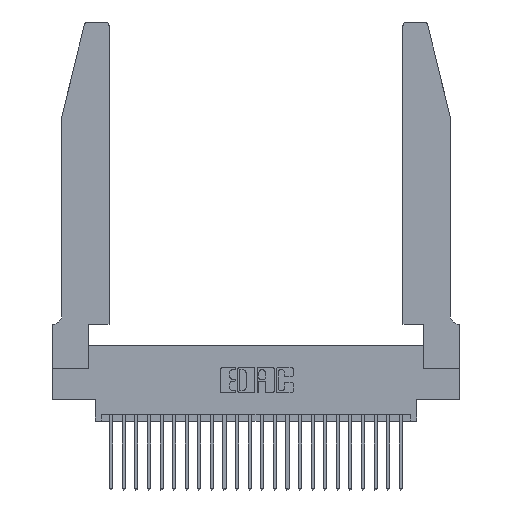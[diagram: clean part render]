
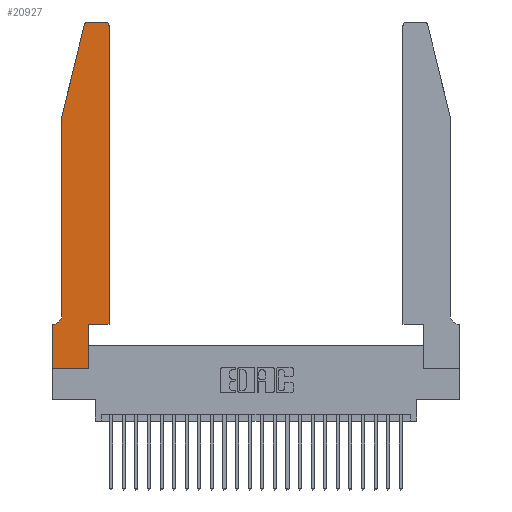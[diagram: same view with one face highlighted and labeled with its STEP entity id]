
A CAD part, top view. The second image highlights one B-rep face of the part: STEP entity #20927.
In plain terms, the highlighted planar face has unit normal (0, 0, 1).
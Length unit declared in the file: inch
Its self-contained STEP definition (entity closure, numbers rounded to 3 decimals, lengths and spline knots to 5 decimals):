
#40 = DIRECTION ( 'NONE',  ( 1., 0., 0. ) ) ;
#59 = EDGE_CURVE ( 'NONE', #6156, #24500, #25750, .T. ) ;
#77 = CARTESIAN_POINT ( 'NONE',  ( 0.2865, 0.35, 0.37 ) ) ;
#344 = DIRECTION ( 'NONE',  ( 0., 1., 0. ) ) ;
#555 = ORIENTED_EDGE ( 'NONE', *, *, #59, .T. ) ;
#828 = VERTEX_POINT ( 'NONE', #5476 ) ;
#865 = AXIS2_PLACEMENT_3D ( 'NONE', #5088, #19230, #7171 ) ;
#963 = VERTEX_POINT ( 'NONE', #14383 ) ;
#1056 = ORIENTED_EDGE ( 'NONE', *, *, #15632, .T. ) ;
#1144 = VECTOR ( 'NONE', #11737, 39.37008 ) ;
#1165 = LINE ( 'NONE', #24578, #11424 ) ;
#1598 = EDGE_CURVE ( 'NONE', #7132, #828, #25560, .T. ) ;
#1786 = VECTOR ( 'NONE', #26148, 39.37008 ) ;
#2011 = CARTESIAN_POINT ( 'NONE',  ( 0.0755, 2., 0.37 ) ) ;
#2216 = ORIENTED_EDGE ( 'NONE', *, *, #18495, .T. ) ;
#3064 = CARTESIAN_POINT ( 'NONE',  ( 0.284, 2.75, 0.37 ) ) ;
#3871 = EDGE_CURVE ( 'NONE', #4540, #17209, #17998, .T. ) ;
#3935 = CARTESIAN_POINT ( 'NONE',  ( 0., 0.35, 0.37 ) ) ;
#3973 = ORIENTED_EDGE ( 'NONE', *, *, #9391, .T. ) ;
#4165 = VERTEX_POINT ( 'NONE', #3064 ) ;
#4263 = FACE_OUTER_BOUND ( 'NONE', #11685, .T. ) ;
#4540 = VERTEX_POINT ( 'NONE', #16641 ) ;
#4904 = LINE ( 'NONE', #23751, #15704 ) ;
#4989 = CARTESIAN_POINT ( 'NONE',  ( 0.4205, 2.72, 0.37 ) ) ;
#5088 = CARTESIAN_POINT ( 'NONE',  ( 0.0055, 0.42, 0.37 ) ) ;
#5476 = CARTESIAN_POINT ( 'NONE',  ( 0.4505, 0.35, 0.37 ) ) ;
#5814 = CARTESIAN_POINT ( 'NONE',  ( 0.2865, 0.35, 0.37 ) ) ;
#5898 = CIRCLE ( 'NONE', #865, 0.07 ) ;
#6156 = VERTEX_POINT ( 'NONE', #20786 ) ;
#6157 = VECTOR ( 'NONE', #11279, 39.37008 ) ;
#6545 = ORIENTED_EDGE ( 'NONE', *, *, #12373, .T. ) ;
#6580 = CARTESIAN_POINT ( 'NONE',  ( 0.0755, 0.42, 0.37 ) ) ;
#6770 = CARTESIAN_POINT ( 'NONE',  ( 0.0755, 2., 0.37 ) ) ;
#7082 = DIRECTION ( 'NONE',  ( 1., 0., 0. ) ) ;
#7125 = DIRECTION ( 'NONE',  ( 0., -1., 0. ) ) ;
#7132 = VERTEX_POINT ( 'NONE', #5814 ) ;
#7171 = DIRECTION ( 'NONE',  ( -1., 0., 0. ) ) ;
#7300 = EDGE_CURVE ( 'NONE', #4165, #4540, #15929, .T. ) ;
#7545 = ORIENTED_EDGE ( 'NONE', *, *, #11584, .T. ) ;
#7758 = DIRECTION ( 'NONE',  ( -1., 0., 0. ) ) ;
#7965 = CARTESIAN_POINT ( 'NONE',  ( 0.4505, 0.35, 0.37 ) ) ;
#8143 = CARTESIAN_POINT ( 'NONE',  ( 0., 0., 0.37 ) ) ;
#8240 = ORIENTED_EDGE ( 'NONE', *, *, #1598, .T. ) ;
#8410 = DIRECTION ( 'NONE',  ( 0., 0., 1. ) ) ;
#8808 = VERTEX_POINT ( 'NONE', #15715 ) ;
#9036 = EDGE_CURVE ( 'NONE', #24500, #7132, #14910, .T. ) ;
#9258 = CARTESIAN_POINT ( 'NONE',  ( 0.2605, 2.75, 0.37 ) ) ;
#9391 = EDGE_CURVE ( 'NONE', #22460, #6156, #22685, .T. ) ;
#9903 = AXIS2_PLACEMENT_3D ( 'NONE', #20460, #8410, #22458 ) ;
#10025 = DIRECTION ( 'NONE',  ( 1., 0., 0. ) ) ;
#10163 = VECTOR ( 'NONE', #14414, 39.37008 ) ;
#11210 = CARTESIAN_POINT ( 'NONE',  ( 0.0755, 2., 0.37 ) ) ;
#11279 = DIRECTION ( 'NONE',  ( -1., 0., 0. ) ) ;
#11424 = VECTOR ( 'NONE', #344, 39.37008 ) ;
#11584 = EDGE_CURVE ( 'NONE', #19014, #8808, #5898, .T. ) ;
#11685 = EDGE_LOOP ( 'NONE', ( #14096, #15001, #23433, #1056, #7545, #6545, #3973, #555, #21401, #8240, #13299, #2216 ) ) ;
#11737 = DIRECTION ( 'NONE',  ( 0., -1., 0. ) ) ;
#12262 = LINE ( 'NONE', #11210, #22262 ) ;
#12373 = EDGE_CURVE ( 'NONE', #8808, #22460, #4904, .T. ) ;
#12774 = EDGE_CURVE ( 'NONE', #963, #4165, #16946, .T. ) ;
#13299 = ORIENTED_EDGE ( 'NONE', *, *, #24487, .T. ) ;
#14096 = ORIENTED_EDGE ( 'NONE', *, *, #12774, .T. ) ;
#14207 = DIRECTION ( 'NONE',  ( 1., 0., 0. ) ) ;
#14383 = CARTESIAN_POINT ( 'NONE',  ( 0.4205, 2.75, 0.37 ) ) ;
#14414 = DIRECTION ( 'NONE',  ( 0., 1., 0. ) ) ;
#14910 = LINE ( 'NONE', #77, #10163 ) ;
#15001 = ORIENTED_EDGE ( 'NONE', *, *, #7300, .T. ) ;
#15632 = EDGE_CURVE ( 'NONE', #17209, #19014, #12262, .T. ) ;
#15704 = VECTOR ( 'NONE', #7758, 39.37008 ) ;
#15715 = CARTESIAN_POINT ( 'NONE',  ( 0.0055, 0.35, 0.37 ) ) ;
#15853 = AXIS2_PLACEMENT_3D ( 'NONE', #3935, #26097, #14207 ) ;
#15929 = CIRCLE ( 'NONE', #9903, 0.03 ) ;
#15949 = VERTEX_POINT ( 'NONE', #22316 ) ;
#16048 = CARTESIAN_POINT ( 'NONE',  ( 0., 0.35, 0.37 ) ) ;
#16641 = CARTESIAN_POINT ( 'NONE',  ( 0.25487, 2.72718, 0.37 ) ) ;
#16946 = LINE ( 'NONE', #9258, #6157 ) ;
#17209 = VERTEX_POINT ( 'NONE', #6770 ) ;
#17998 = LINE ( 'NONE', #2011, #1786 ) ;
#18000 = AXIS2_PLACEMENT_3D ( 'NONE', #4989, #19143, #7082 ) ;
#18495 = EDGE_CURVE ( 'NONE', #15949, #963, #19623, .T. ) ;
#19014 = VERTEX_POINT ( 'NONE', #6580 ) ;
#19143 = DIRECTION ( 'NONE',  ( 0., 0., 1. ) ) ;
#19230 = DIRECTION ( 'NONE',  ( 0., 0., -1. ) ) ;
#19623 = CIRCLE ( 'NONE', #18000, 0.03 ) ;
#20120 = PLANE ( 'NONE',  #15853 ) ;
#20296 = VECTOR ( 'NONE', #40, 39.37008 ) ;
#20460 = CARTESIAN_POINT ( 'NONE',  ( 0.284, 2.72, 0.37 ) ) ;
#20487 = VECTOR ( 'NONE', #10025, 39.37008 ) ;
#20675 = CARTESIAN_POINT ( 'NONE',  ( 0.2865, 0., 0.37 ) ) ;
#20786 = CARTESIAN_POINT ( 'NONE',  ( 0., 0., 0.37 ) ) ;
#20927 = ADVANCED_FACE ( 'NONE', ( #4263 ), #20120, .T. ) ;
#21401 = ORIENTED_EDGE ( 'NONE', *, *, #9036, .T. ) ;
#21731 = CARTESIAN_POINT ( 'NONE',  ( 0., 0., 0.37 ) ) ;
#22262 = VECTOR ( 'NONE', #7125, 39.37008 ) ;
#22316 = CARTESIAN_POINT ( 'NONE',  ( 0.4505, 2.72, 0.37 ) ) ;
#22458 = DIRECTION ( 'NONE',  ( 1., 0., 0. ) ) ;
#22460 = VERTEX_POINT ( 'NONE', #16048 ) ;
#22685 = LINE ( 'NONE', #21731, #1144 ) ;
#23433 = ORIENTED_EDGE ( 'NONE', *, *, #3871, .T. ) ;
#23751 = CARTESIAN_POINT ( 'NONE',  ( 0.0755, 0.35, 0.37 ) ) ;
#24487 = EDGE_CURVE ( 'NONE', #828, #15949, #1165, .T. ) ;
#24500 = VERTEX_POINT ( 'NONE', #20675 ) ;
#24578 = CARTESIAN_POINT ( 'NONE',  ( 0.4505, 0.35, 0.37 ) ) ;
#25560 = LINE ( 'NONE', #7965, #20296 ) ;
#25750 = LINE ( 'NONE', #8143, #20487 ) ;
#26097 = DIRECTION ( 'NONE',  ( 0., 0., 1. ) ) ;
#26148 = DIRECTION ( 'NONE',  ( -0.239, -0.971, 0. ) ) ;
